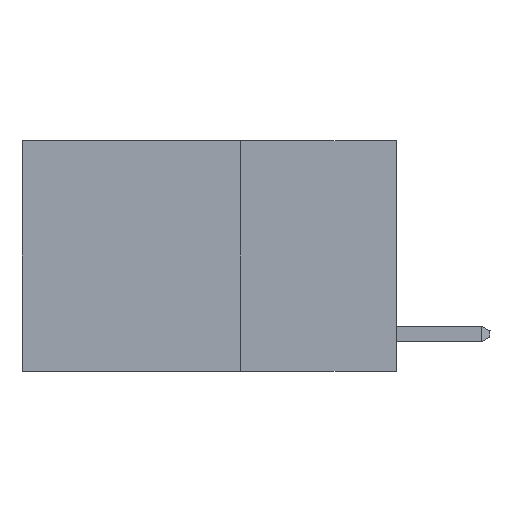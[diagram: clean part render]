
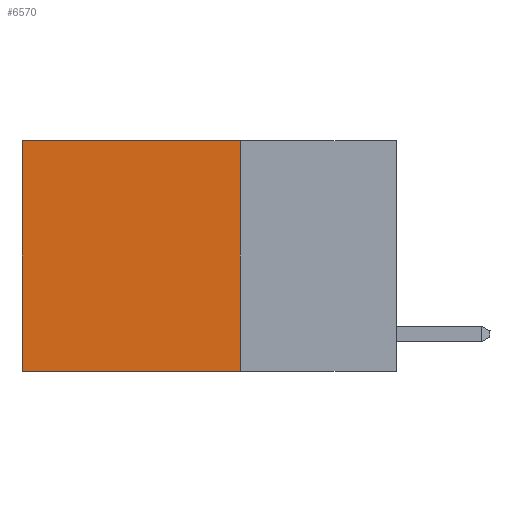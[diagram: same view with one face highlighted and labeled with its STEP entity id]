
A CAD part, left-side view. The second image highlights one B-rep face of the part: STEP entity #6570.
In plain terms, the highlighted planar face has unit normal (-1, 0, 0).
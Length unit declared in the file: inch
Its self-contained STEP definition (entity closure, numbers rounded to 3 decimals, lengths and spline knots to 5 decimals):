
#36 = EDGE_LOOP ( 'NONE', ( #12109, #14299, #7811, #3795 ) ) ;
#356 = DIRECTION ( 'NONE',  ( 0., 0., -1. ) ) ;
#574 = CARTESIAN_POINT ( 'NONE',  ( 0.2625, 0.25, -0.37 ) ) ;
#677 = VECTOR ( 'NONE', #2932, 39.37008 ) ;
#1109 = VECTOR ( 'NONE', #2907, 39.37008 ) ;
#1127 = DIRECTION ( 'NONE',  ( 1., 0., 0. ) ) ;
#2907 = DIRECTION ( 'NONE',  ( 0., 1., 0. ) ) ;
#2932 = DIRECTION ( 'NONE',  ( 0., 0., -1. ) ) ;
#3406 = VERTEX_POINT ( 'NONE', #10705 ) ;
#3795 = ORIENTED_EDGE ( 'NONE', *, *, #8171, .T. ) ;
#4007 = VERTEX_POINT ( 'NONE', #12251 ) ;
#4555 = VERTEX_POINT ( 'NONE', #10421 ) ;
#4638 = CARTESIAN_POINT ( 'NONE',  ( 0.2625, 0.25, 0. ) ) ;
#4785 = LINE ( 'NONE', #4638, #13113 ) ;
#5999 = AXIS2_PLACEMENT_3D ( 'NONE', #12571, #1127, #9996 ) ;
#6570 = ADVANCED_FACE ( 'NONE', ( #8956 ), #14821, .F. ) ;
#7811 = ORIENTED_EDGE ( 'NONE', *, *, #13343, .F. ) ;
#8091 = CARTESIAN_POINT ( 'NONE',  ( 0.2625, 0.25, 0. ) ) ;
#8171 = EDGE_CURVE ( 'NONE', #4007, #4555, #4785, .T. ) ;
#8318 = LINE ( 'NONE', #8091, #10297 ) ;
#8956 = FACE_OUTER_BOUND ( 'NONE', #36, .T. ) ;
#9182 = EDGE_CURVE ( 'NONE', #3406, #12969, #9590, .T. ) ;
#9444 = CARTESIAN_POINT ( 'NONE',  ( 0.2625, 0.6, -0.37 ) ) ;
#9590 = LINE ( 'NONE', #574, #1109 ) ;
#9977 = LINE ( 'NONE', #13388, #677 ) ;
#9996 = DIRECTION ( 'NONE',  ( 0., 0., -1. ) ) ;
#10297 = VECTOR ( 'NONE', #356, 39.37008 ) ;
#10421 = CARTESIAN_POINT ( 'NONE',  ( 0.2625, 0.6, 0. ) ) ;
#10497 = DIRECTION ( 'NONE',  ( 0., 1., 0. ) ) ;
#10688 = EDGE_CURVE ( 'NONE', #4555, #12969, #9977, .T. ) ;
#10705 = CARTESIAN_POINT ( 'NONE',  ( 0.2625, 0.25, -0.37 ) ) ;
#12109 = ORIENTED_EDGE ( 'NONE', *, *, #10688, .T. ) ;
#12251 = CARTESIAN_POINT ( 'NONE',  ( 0.2625, 0.25, 0. ) ) ;
#12571 = CARTESIAN_POINT ( 'NONE',  ( 0.2625, 0.25, 0. ) ) ;
#12969 = VERTEX_POINT ( 'NONE', #9444 ) ;
#13113 = VECTOR ( 'NONE', #10497, 39.37008 ) ;
#13343 = EDGE_CURVE ( 'NONE', #4007, #3406, #8318, .T. ) ;
#13388 = CARTESIAN_POINT ( 'NONE',  ( 0.2625, 0.6, 0. ) ) ;
#14299 = ORIENTED_EDGE ( 'NONE', *, *, #9182, .F. ) ;
#14821 = PLANE ( 'NONE',  #5999 ) ;
